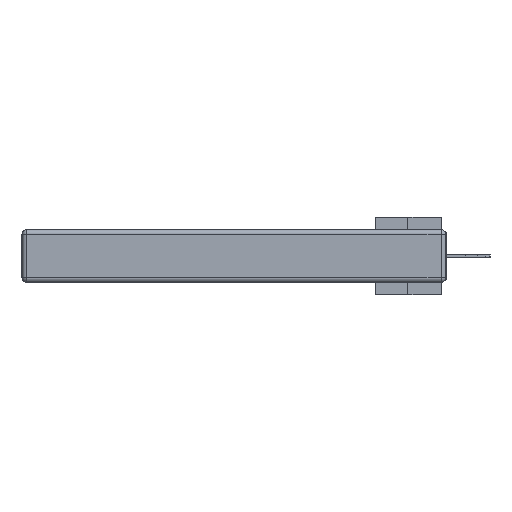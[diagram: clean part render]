
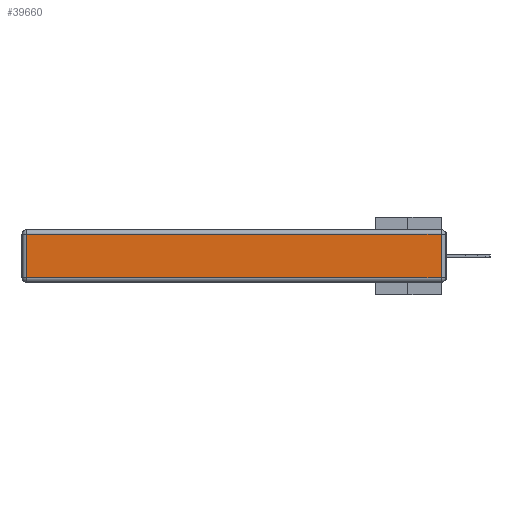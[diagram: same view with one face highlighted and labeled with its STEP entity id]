
A CAD part, left-side view. The second image highlights one B-rep face of the part: STEP entity #39660.
In plain terms, the highlighted planar face has unit normal (-1, 0, 0).
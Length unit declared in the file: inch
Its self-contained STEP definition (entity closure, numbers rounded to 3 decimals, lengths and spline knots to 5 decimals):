
#1267 = VECTOR ( 'NONE', #40330, 39.37008 ) ;
#2139 = VECTOR ( 'NONE', #36385, 39.37008 ) ;
#3737 = EDGE_LOOP ( 'NONE', ( #23583, #27494, #27023, #34198 ) ) ;
#4833 = CARTESIAN_POINT ( 'NONE',  ( 0., 2.72, -0.343 ) ) ;
#5141 = LINE ( 'NONE', #24011, #2139 ) ;
#5324 = CARTESIAN_POINT ( 'NONE',  ( 0., 0., -0.343 ) ) ;
#5819 = VERTEX_POINT ( 'NONE', #10332 ) ;
#6078 = VERTEX_POINT ( 'NONE', #8916 ) ;
#6681 = CARTESIAN_POINT ( 'NONE',  ( 0., 0.03, -0.03 ) ) ;
#8516 = DIRECTION ( 'NONE',  ( 0., 0., 1. ) ) ;
#8916 = CARTESIAN_POINT ( 'NONE',  ( 0., 2.72, -0.313 ) ) ;
#10080 = VECTOR ( 'NONE', #20382, 39.37008 ) ;
#10332 = CARTESIAN_POINT ( 'NONE',  ( 0., 0.03, -0.313 ) ) ;
#11529 = PLANE ( 'NONE',  #29681 ) ;
#13329 = EDGE_CURVE ( 'NONE', #40202, #6078, #26516, .T. ) ;
#16120 = EDGE_CURVE ( 'NONE', #20412, #40202, #18107, .T. ) ;
#17129 = CARTESIAN_POINT ( 'NONE',  ( 0., 2.75, -0.03 ) ) ;
#18107 = LINE ( 'NONE', #17129, #33648 ) ;
#20233 = DIRECTION ( 'NONE',  ( 0., 1., 0. ) ) ;
#20382 = DIRECTION ( 'NONE',  ( 0., 0., -1. ) ) ;
#20412 = VERTEX_POINT ( 'NONE', #6681 ) ;
#23583 = ORIENTED_EDGE ( 'NONE', *, *, #26636, .T. ) ;
#24011 = CARTESIAN_POINT ( 'NONE',  ( 0., 0.03, -0.343 ) ) ;
#25228 = LINE ( 'NONE', #37337, #1267 ) ;
#26516 = LINE ( 'NONE', #4833, #10080 ) ;
#26636 = EDGE_CURVE ( 'NONE', #6078, #5819, #25228, .T. ) ;
#27023 = ORIENTED_EDGE ( 'NONE', *, *, #16120, .T. ) ;
#27088 = DIRECTION ( 'NONE',  ( -1., 0., 0. ) ) ;
#27494 = ORIENTED_EDGE ( 'NONE', *, *, #36352, .T. ) ;
#29681 = AXIS2_PLACEMENT_3D ( 'NONE', #5324, #27088, #8516 ) ;
#29782 = CARTESIAN_POINT ( 'NONE',  ( 0., 2.72, -0.03 ) ) ;
#33648 = VECTOR ( 'NONE', #20233, 39.37008 ) ;
#34198 = ORIENTED_EDGE ( 'NONE', *, *, #13329, .T. ) ;
#34555 = FACE_OUTER_BOUND ( 'NONE', #3737, .T. ) ;
#36352 = EDGE_CURVE ( 'NONE', #5819, #20412, #5141, .T. ) ;
#36385 = DIRECTION ( 'NONE',  ( 0., 0., 1. ) ) ;
#37337 = CARTESIAN_POINT ( 'NONE',  ( 0., 0., -0.313 ) ) ;
#39660 = ADVANCED_FACE ( 'NONE', ( #34555 ), #11529, .T. ) ;
#40202 = VERTEX_POINT ( 'NONE', #29782 ) ;
#40330 = DIRECTION ( 'NONE',  ( 0., -1., 0. ) ) ;
